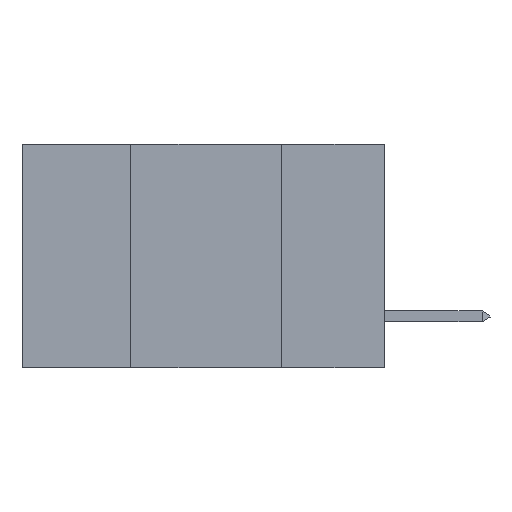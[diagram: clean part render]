
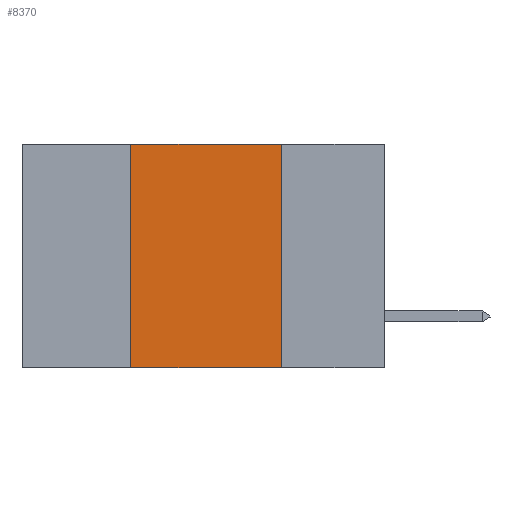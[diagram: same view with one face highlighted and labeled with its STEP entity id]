
A CAD part, left-side view. The second image highlights one B-rep face of the part: STEP entity #8370.
In plain terms, the highlighted planar face has unit normal (-1, 0, 0).
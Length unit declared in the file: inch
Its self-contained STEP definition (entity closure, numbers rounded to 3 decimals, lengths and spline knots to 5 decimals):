
#835 = ORIENTED_EDGE ( 'NONE', *, *, #21353, .F. ) ;
#1398 = DIRECTION ( 'NONE',  ( 0., 0., -1. ) ) ;
#3581 = LINE ( 'NONE', #21414, #17068 ) ;
#4024 = EDGE_CURVE ( 'NONE', #19191, #6195, #3581, .T. ) ;
#6153 = DIRECTION ( 'NONE',  ( 0., -1., 0. ) ) ;
#6195 = VERTEX_POINT ( 'NONE', #12364 ) ;
#6999 = CARTESIAN_POINT ( 'NONE',  ( 0., 0.42, 0. ) ) ;
#7024 = PLANE ( 'NONE',  #14247 ) ;
#7804 = LINE ( 'NONE', #16542, #13972 ) ;
#8370 = ADVANCED_FACE ( 'NONE', ( #18886 ), #7024, .F. ) ;
#8431 = CARTESIAN_POINT ( 'NONE',  ( 0., 0.42, -0.37 ) ) ;
#9123 = EDGE_CURVE ( 'NONE', #19191, #9262, #11474, .T. ) ;
#9172 = CARTESIAN_POINT ( 'NONE',  ( 0., 0.6, 0. ) ) ;
#9262 = VERTEX_POINT ( 'NONE', #14088 ) ;
#9432 = VERTEX_POINT ( 'NONE', #23346 ) ;
#9841 = DIRECTION ( 'NONE',  ( 0., 0., 1. ) ) ;
#10425 = LINE ( 'NONE', #9172, #11597 ) ;
#11227 = ORIENTED_EDGE ( 'NONE', *, *, #20769, .F. ) ;
#11474 = LINE ( 'NONE', #6999, #13254 ) ;
#11597 = VECTOR ( 'NONE', #16718, 39.37008 ) ;
#12364 = CARTESIAN_POINT ( 'NONE',  ( 0., 0.17, -0.37 ) ) ;
#12489 = ORIENTED_EDGE ( 'NONE', *, *, #4024, .T. ) ;
#13254 = VECTOR ( 'NONE', #9841, 39.37008 ) ;
#13972 = VECTOR ( 'NONE', #22031, 39.37008 ) ;
#14088 = CARTESIAN_POINT ( 'NONE',  ( 0., 0.42, 0. ) ) ;
#14247 = AXIS2_PLACEMENT_3D ( 'NONE', #16491, #14442, #1398 ) ;
#14442 = DIRECTION ( 'NONE',  ( 1., 0., 0. ) ) ;
#16491 = CARTESIAN_POINT ( 'NONE',  ( 0., 0.6, 0. ) ) ;
#16542 = CARTESIAN_POINT ( 'NONE',  ( 0., 0.17, 0. ) ) ;
#16718 = DIRECTION ( 'NONE',  ( 0., -1., 0. ) ) ;
#16792 = EDGE_LOOP ( 'NONE', ( #11227, #835, #20628, #12489 ) ) ;
#17068 = VECTOR ( 'NONE', #6153, 39.37008 ) ;
#18886 = FACE_OUTER_BOUND ( 'NONE', #16792, .T. ) ;
#19191 = VERTEX_POINT ( 'NONE', #8431 ) ;
#20628 = ORIENTED_EDGE ( 'NONE', *, *, #9123, .F. ) ;
#20769 = EDGE_CURVE ( 'NONE', #9432, #6195, #7804, .T. ) ;
#21353 = EDGE_CURVE ( 'NONE', #9262, #9432, #10425, .T. ) ;
#21414 = CARTESIAN_POINT ( 'NONE',  ( 0., 0.6, -0.37 ) ) ;
#22031 = DIRECTION ( 'NONE',  ( 0., 0., -1. ) ) ;
#23346 = CARTESIAN_POINT ( 'NONE',  ( 0., 0.17, 0. ) ) ;
